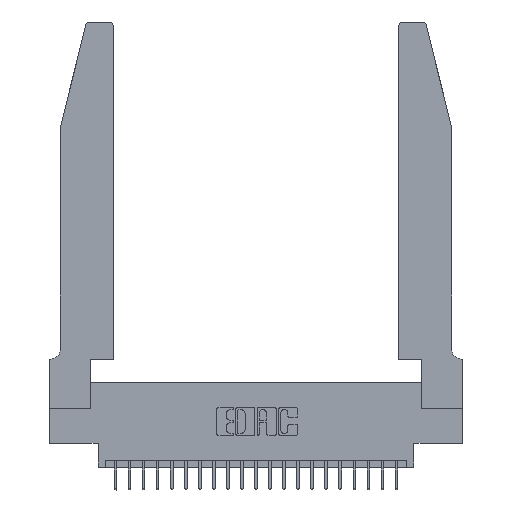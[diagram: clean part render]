
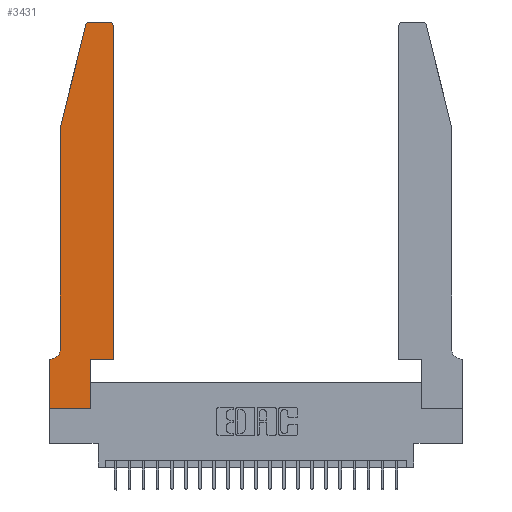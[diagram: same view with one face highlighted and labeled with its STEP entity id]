
A CAD part, top view. The second image highlights one B-rep face of the part: STEP entity #3431.
In plain terms, the highlighted planar face has unit normal (0, 0, 1).
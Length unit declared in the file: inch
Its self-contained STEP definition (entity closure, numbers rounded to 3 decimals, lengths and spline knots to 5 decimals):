
#98 = ORIENTED_EDGE ( 'NONE', *, *, #1568, .T. ) ;
#267 = DIRECTION ( 'NONE',  ( 0., -1., 0. ) ) ;
#759 = DIRECTION ( 'NONE',  ( 0., 0., 1. ) ) ;
#928 = VERTEX_POINT ( 'NONE', #15770 ) ;
#1281 = ORIENTED_EDGE ( 'NONE', *, *, #2043, .T. ) ;
#1377 = LINE ( 'NONE', #7125, #18399 ) ;
#1414 = DIRECTION ( 'NONE',  ( 0., 1., 0. ) ) ;
#1433 = DIRECTION ( 'NONE',  ( 1., 0., 0. ) ) ;
#1568 = EDGE_CURVE ( 'NONE', #5463, #928, #23044, .T. ) ;
#1605 = CARTESIAN_POINT ( 'NONE',  ( 0.284, 2.72, 0.37 ) ) ;
#1703 = CARTESIAN_POINT ( 'NONE',  ( 0.284, 2.75, 0.37 ) ) ;
#2043 = EDGE_CURVE ( 'NONE', #10299, #22059, #12765, .T. ) ;
#2049 = ORIENTED_EDGE ( 'NONE', *, *, #22390, .T. ) ;
#2315 = DIRECTION ( 'NONE',  ( 0., -1., 0. ) ) ;
#2385 = DIRECTION ( 'NONE',  ( 1., 0., 0. ) ) ;
#3190 = ORIENTED_EDGE ( 'NONE', *, *, #21287, .T. ) ;
#3431 = ADVANCED_FACE ( 'NONE', ( #22590 ), #17937, .T. ) ;
#3504 = DIRECTION ( 'NONE',  ( -1., 0., 0. ) ) ;
#4065 = DIRECTION ( 'NONE',  ( -1., 0., 0. ) ) ;
#4081 = CIRCLE ( 'NONE', #14476, 0.03 ) ;
#4193 = CARTESIAN_POINT ( 'NONE',  ( 0.0055, 0.35, 0.37 ) ) ;
#4717 = CARTESIAN_POINT ( 'NONE',  ( 0., 0.35, 0.37 ) ) ;
#4838 = ORIENTED_EDGE ( 'NONE', *, *, #10366, .T. ) ;
#4893 = VERTEX_POINT ( 'NONE', #10129 ) ;
#5133 = CARTESIAN_POINT ( 'NONE',  ( 0.2605, 2.75, 0.37 ) ) ;
#5260 = VECTOR ( 'NONE', #1414, 39.37008 ) ;
#5368 = AXIS2_PLACEMENT_3D ( 'NONE', #4717, #7593, #2385 ) ;
#5406 = EDGE_CURVE ( 'NONE', #6787, #14734, #19901, .T. ) ;
#5463 = VERTEX_POINT ( 'NONE', #4193 ) ;
#6149 = CARTESIAN_POINT ( 'NONE',  ( 0.4505, 0.35, 0.37 ) ) ;
#6787 = VERTEX_POINT ( 'NONE', #17366 ) ;
#7125 = CARTESIAN_POINT ( 'NONE',  ( 0.0755, 2., 0.37 ) ) ;
#7169 = EDGE_CURVE ( 'NONE', #22059, #23757, #14539, .T. ) ;
#7593 = DIRECTION ( 'NONE',  ( 0., 0., 1. ) ) ;
#8143 = CARTESIAN_POINT ( 'NONE',  ( 0., 0., 0.37 ) ) ;
#8308 = CARTESIAN_POINT ( 'NONE',  ( 0., 0., 0.37 ) ) ;
#9299 = VECTOR ( 'NONE', #267, 39.37008 ) ;
#9752 = DIRECTION ( 'NONE',  ( 1., 0., 0. ) ) ;
#10081 = ORIENTED_EDGE ( 'NONE', *, *, #20096, .T. ) ;
#10125 = CIRCLE ( 'NONE', #15908, 0.07 ) ;
#10129 = CARTESIAN_POINT ( 'NONE',  ( 0.0755, 0.42, 0.37 ) ) ;
#10282 = EDGE_CURVE ( 'NONE', #23757, #6787, #16336, .T. ) ;
#10299 = VERTEX_POINT ( 'NONE', #8143 ) ;
#10366 = EDGE_CURVE ( 'NONE', #4893, #5463, #10125, .T. ) ;
#10414 = AXIS2_PLACEMENT_3D ( 'NONE', #1605, #22061, #1433 ) ;
#10427 = VECTOR ( 'NONE', #19794, 39.37008 ) ;
#10634 = EDGE_LOOP ( 'NONE', ( #19045, #2049, #12600, #3190, #4838, #98, #19927, #1281, #23039, #14069, #16485, #10081 ) ) ;
#10655 = EDGE_CURVE ( 'NONE', #11736, #15673, #21846, .T. ) ;
#10864 = CARTESIAN_POINT ( 'NONE',  ( 0.2865, 0.35, 0.37 ) ) ;
#11440 = CARTESIAN_POINT ( 'NONE',  ( 0.0755, 2., 0.37 ) ) ;
#11736 = VERTEX_POINT ( 'NONE', #12953 ) ;
#12149 = CARTESIAN_POINT ( 'NONE',  ( 0.4205, 2.72, 0.37 ) ) ;
#12188 = CIRCLE ( 'NONE', #10414, 0.03 ) ;
#12224 = CARTESIAN_POINT ( 'NONE',  ( 0.2865, 0.35, 0.37 ) ) ;
#12504 = VECTOR ( 'NONE', #4065, 39.37008 ) ;
#12600 = ORIENTED_EDGE ( 'NONE', *, *, #16240, .T. ) ;
#12671 = CARTESIAN_POINT ( 'NONE',  ( 0.0055, 0.42, 0.37 ) ) ;
#12765 = LINE ( 'NONE', #15139, #23903 ) ;
#12840 = LINE ( 'NONE', #11440, #9299 ) ;
#12953 = CARTESIAN_POINT ( 'NONE',  ( 0.4205, 2.75, 0.37 ) ) ;
#13018 = DIRECTION ( 'NONE',  ( -0.239, -0.971, 0. ) ) ;
#13700 = CARTESIAN_POINT ( 'NONE',  ( 0.25487, 2.72718, 0.37 ) ) ;
#14069 = ORIENTED_EDGE ( 'NONE', *, *, #10282, .T. ) ;
#14228 = CARTESIAN_POINT ( 'NONE',  ( 0.0755, 2., 0.37 ) ) ;
#14256 = VECTOR ( 'NONE', #9752, 39.37008 ) ;
#14476 = AXIS2_PLACEMENT_3D ( 'NONE', #12149, #759, #19776 ) ;
#14539 = LINE ( 'NONE', #12224, #22153 ) ;
#14734 = VERTEX_POINT ( 'NONE', #16660 ) ;
#15139 = CARTESIAN_POINT ( 'NONE',  ( 0., 0., 0.37 ) ) ;
#15189 = CARTESIAN_POINT ( 'NONE',  ( 0.0755, 0.35, 0.37 ) ) ;
#15673 = VERTEX_POINT ( 'NONE', #1703 ) ;
#15770 = CARTESIAN_POINT ( 'NONE',  ( 0., 0.35, 0.37 ) ) ;
#15908 = AXIS2_PLACEMENT_3D ( 'NONE', #12671, #20208, #3504 ) ;
#16005 = EDGE_CURVE ( 'NONE', #928, #10299, #22476, .T. ) ;
#16240 = EDGE_CURVE ( 'NONE', #24016, #19736, #1377, .T. ) ;
#16336 = LINE ( 'NONE', #6149, #14256 ) ;
#16348 = VECTOR ( 'NONE', #2315, 39.37008 ) ;
#16485 = ORIENTED_EDGE ( 'NONE', *, *, #5406, .T. ) ;
#16660 = CARTESIAN_POINT ( 'NONE',  ( 0.4505, 2.72, 0.37 ) ) ;
#16734 = DIRECTION ( 'NONE',  ( 1., 0., 0. ) ) ;
#16882 = CARTESIAN_POINT ( 'NONE',  ( 0.4505, 0.35, 0.37 ) ) ;
#17366 = CARTESIAN_POINT ( 'NONE',  ( 0.4505, 0.35, 0.37 ) ) ;
#17937 = PLANE ( 'NONE',  #5368 ) ;
#18399 = VECTOR ( 'NONE', #13018, 39.37008 ) ;
#19045 = ORIENTED_EDGE ( 'NONE', *, *, #10655, .T. ) ;
#19736 = VERTEX_POINT ( 'NONE', #14228 ) ;
#19776 = DIRECTION ( 'NONE',  ( 1., 0., 0. ) ) ;
#19794 = DIRECTION ( 'NONE',  ( -1., 0., 0. ) ) ;
#19901 = LINE ( 'NONE', #16882, #5260 ) ;
#19927 = ORIENTED_EDGE ( 'NONE', *, *, #16005, .T. ) ;
#20096 = EDGE_CURVE ( 'NONE', #14734, #11736, #4081, .T. ) ;
#20134 = DIRECTION ( 'NONE',  ( 0., 1., 0. ) ) ;
#20208 = DIRECTION ( 'NONE',  ( 0., 0., -1. ) ) ;
#21287 = EDGE_CURVE ( 'NONE', #19736, #4893, #12840, .T. ) ;
#21846 = LINE ( 'NONE', #5133, #10427 ) ;
#22059 = VERTEX_POINT ( 'NONE', #23285 ) ;
#22061 = DIRECTION ( 'NONE',  ( 0., 0., 1. ) ) ;
#22153 = VECTOR ( 'NONE', #20134, 39.37008 ) ;
#22390 = EDGE_CURVE ( 'NONE', #15673, #24016, #12188, .T. ) ;
#22476 = LINE ( 'NONE', #8308, #16348 ) ;
#22590 = FACE_OUTER_BOUND ( 'NONE', #10634, .T. ) ;
#23039 = ORIENTED_EDGE ( 'NONE', *, *, #7169, .T. ) ;
#23044 = LINE ( 'NONE', #15189, #12504 ) ;
#23285 = CARTESIAN_POINT ( 'NONE',  ( 0.2865, 0., 0.37 ) ) ;
#23757 = VERTEX_POINT ( 'NONE', #10864 ) ;
#23903 = VECTOR ( 'NONE', #16734, 39.37008 ) ;
#24016 = VERTEX_POINT ( 'NONE', #13700 ) ;
